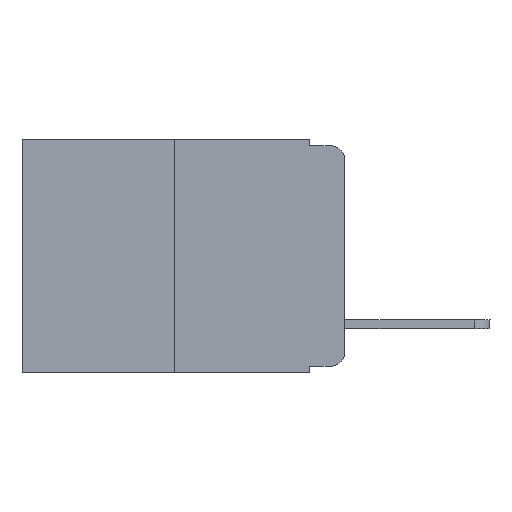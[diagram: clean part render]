
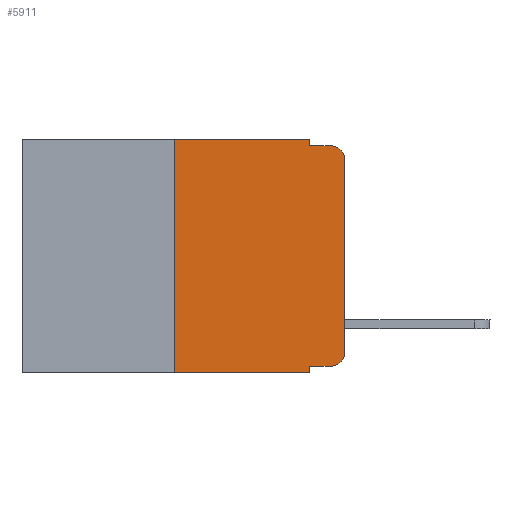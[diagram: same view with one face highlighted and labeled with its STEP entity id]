
A CAD part, left-side view. The second image highlights one B-rep face of the part: STEP entity #5911.
In plain terms, the highlighted planar face has unit normal (-1, 0, 0).
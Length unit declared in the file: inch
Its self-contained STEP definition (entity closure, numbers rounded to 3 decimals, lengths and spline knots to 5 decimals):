
#276 = EDGE_CURVE ( 'NONE', #9761, #8331, #9257, .T. ) ;
#400 = LINE ( 'NONE', #3320, #4874 ) ;
#403 = EDGE_CURVE ( 'NONE', #9929, #1436, #1438, .T. ) ;
#470 = CIRCLE ( 'NONE', #8765, 0.02 ) ;
#558 = EDGE_CURVE ( 'NONE', #2085, #9761, #470, .T. ) ;
#582 = VERTEX_POINT ( 'NONE', #11100 ) ;
#621 = CARTESIAN_POINT ( 'NONE',  ( 0., 0.25, 0. ) ) ;
#785 = AXIS2_PLACEMENT_3D ( 'NONE', #1922, #5697, #9461 ) ;
#867 = EDGE_CURVE ( 'NONE', #1587, #10772, #5343, .T. ) ;
#919 = DIRECTION ( 'NONE',  ( 0., -1., 0. ) ) ;
#1420 = CARTESIAN_POINT ( 'NONE',  ( 0., 0.02, -0.03 ) ) ;
#1436 = VERTEX_POINT ( 'NONE', #10726 ) ;
#1438 = LINE ( 'NONE', #5167, #6863 ) ;
#1571 = LINE ( 'NONE', #3662, #1949 ) ;
#1587 = VERTEX_POINT ( 'NONE', #9010 ) ;
#1632 = CARTESIAN_POINT ( 'NONE',  ( 0., 0.02, -0.313 ) ) ;
#1808 = CARTESIAN_POINT ( 'NONE',  ( 0., 0., -0.313 ) ) ;
#1860 = LINE ( 'NONE', #5636, #4033 ) ;
#1922 = CARTESIAN_POINT ( 'NONE',  ( 0., 0.473, 0. ) ) ;
#1949 = VECTOR ( 'NONE', #4356, 39.37008 ) ;
#2085 = VERTEX_POINT ( 'NONE', #3665 ) ;
#2093 = ORIENTED_EDGE ( 'NONE', *, *, #8308, .T. ) ;
#2162 = DIRECTION ( 'NONE',  ( 0., 0., -1. ) ) ;
#2482 = DIRECTION ( 'NONE',  ( 0., 0., -1. ) ) ;
#2676 = ORIENTED_EDGE ( 'NONE', *, *, #8798, .F. ) ;
#2782 = LINE ( 'NONE', #4708, #9249 ) ;
#2839 = DIRECTION ( 'NONE',  ( 0., 0., -1. ) ) ;
#2946 = AXIS2_PLACEMENT_3D ( 'NONE', #1420, #5276, #2482 ) ;
#3130 = DIRECTION ( 'NONE',  ( 0., -1., 0. ) ) ;
#3320 = CARTESIAN_POINT ( 'NONE',  ( 0., 0.473, 0. ) ) ;
#3329 = LINE ( 'NONE', #7101, #8685 ) ;
#3350 = CIRCLE ( 'NONE', #2946, 0.02 ) ;
#3431 = DIRECTION ( 'NONE',  ( 0., 0., -1. ) ) ;
#3662 = CARTESIAN_POINT ( 'NONE',  ( 0., 0.473, -0.343 ) ) ;
#3665 = CARTESIAN_POINT ( 'NONE',  ( 0., 0.02, -0.333 ) ) ;
#3875 = ORIENTED_EDGE ( 'NONE', *, *, #558, .T. ) ;
#4033 = VECTOR ( 'NONE', #919, 39.37008 ) ;
#4095 = CARTESIAN_POINT ( 'NONE',  ( 0., 0.25, 0. ) ) ;
#4145 = EDGE_LOOP ( 'NONE', ( #9566, #2093, #7808, #2676, #6607, #5915, #6274, #9832, #5366, #3875 ) ) ;
#4148 = EDGE_CURVE ( 'NONE', #4573, #582, #2782, .T. ) ;
#4356 = DIRECTION ( 'NONE',  ( 0., -1., 0. ) ) ;
#4375 = DIRECTION ( 'NONE',  ( 0., 0., 1. ) ) ;
#4403 = DIRECTION ( 'NONE',  ( 0., 0., 1. ) ) ;
#4573 = VERTEX_POINT ( 'NONE', #10615 ) ;
#4636 = PLANE ( 'NONE',  #785 ) ;
#4708 = CARTESIAN_POINT ( 'NONE',  ( 0., 0.051, 0. ) ) ;
#4874 = VECTOR ( 'NONE', #3130, 39.37008 ) ;
#4876 = EDGE_CURVE ( 'NONE', #1587, #582, #1571, .T. ) ;
#5075 = CARTESIAN_POINT ( 'NONE',  ( 0., 0.051, 0. ) ) ;
#5167 = CARTESIAN_POINT ( 'NONE',  ( 0., 0.051, -0.01 ) ) ;
#5276 = DIRECTION ( 'NONE',  ( -1., 0., 0. ) ) ;
#5343 = LINE ( 'NONE', #621, #7005 ) ;
#5366 = ORIENTED_EDGE ( 'NONE', *, *, #9819, .T. ) ;
#5636 = CARTESIAN_POINT ( 'NONE',  ( 0., 0.051, -0.333 ) ) ;
#5697 = DIRECTION ( 'NONE',  ( 1., 0., 0. ) ) ;
#5911 = ADVANCED_FACE ( 'NONE', ( #10384 ), #4636, .F. ) ;
#5915 = ORIENTED_EDGE ( 'NONE', *, *, #867, .F. ) ;
#6153 = EDGE_CURVE ( 'NONE', #10772, #7994, #400, .T. ) ;
#6274 = ORIENTED_EDGE ( 'NONE', *, *, #4876, .T. ) ;
#6607 = ORIENTED_EDGE ( 'NONE', *, *, #6153, .F. ) ;
#6863 = VECTOR ( 'NONE', #7939, 39.37008 ) ;
#7005 = VECTOR ( 'NONE', #4403, 39.37008 ) ;
#7101 = CARTESIAN_POINT ( 'NONE',  ( 0., 0.051, 0. ) ) ;
#7808 = ORIENTED_EDGE ( 'NONE', *, *, #403, .F. ) ;
#7939 = DIRECTION ( 'NONE',  ( 0., -1., 0. ) ) ;
#7994 = VERTEX_POINT ( 'NONE', #5075 ) ;
#8267 = CARTESIAN_POINT ( 'NONE',  ( 0., 0., 0. ) ) ;
#8308 = EDGE_CURVE ( 'NONE', #8331, #1436, #3350, .T. ) ;
#8313 = DIRECTION ( 'NONE',  ( -1., 0., 0. ) ) ;
#8331 = VERTEX_POINT ( 'NONE', #9905 ) ;
#8685 = VECTOR ( 'NONE', #2162, 39.37008 ) ;
#8765 = AXIS2_PLACEMENT_3D ( 'NONE', #1632, #8313, #3431 ) ;
#8798 = EDGE_CURVE ( 'NONE', #7994, #9929, #3329, .T. ) ;
#9010 = CARTESIAN_POINT ( 'NONE',  ( 0., 0.25, -0.343 ) ) ;
#9249 = VECTOR ( 'NONE', #2839, 39.37008 ) ;
#9257 = LINE ( 'NONE', #8267, #11608 ) ;
#9461 = DIRECTION ( 'NONE',  ( 0., 0., -1. ) ) ;
#9566 = ORIENTED_EDGE ( 'NONE', *, *, #276, .T. ) ;
#9761 = VERTEX_POINT ( 'NONE', #1808 ) ;
#9819 = EDGE_CURVE ( 'NONE', #4573, #2085, #1860, .T. ) ;
#9832 = ORIENTED_EDGE ( 'NONE', *, *, #4148, .F. ) ;
#9905 = CARTESIAN_POINT ( 'NONE',  ( 0., 0., -0.03 ) ) ;
#9929 = VERTEX_POINT ( 'NONE', #11321 ) ;
#10384 = FACE_OUTER_BOUND ( 'NONE', #4145, .T. ) ;
#10615 = CARTESIAN_POINT ( 'NONE',  ( 0., 0.051, -0.333 ) ) ;
#10726 = CARTESIAN_POINT ( 'NONE',  ( 0., 0.02, -0.01 ) ) ;
#10772 = VERTEX_POINT ( 'NONE', #4095 ) ;
#11100 = CARTESIAN_POINT ( 'NONE',  ( 0., 0.051, -0.343 ) ) ;
#11321 = CARTESIAN_POINT ( 'NONE',  ( 0., 0.051, -0.01 ) ) ;
#11608 = VECTOR ( 'NONE', #4375, 39.37008 ) ;
